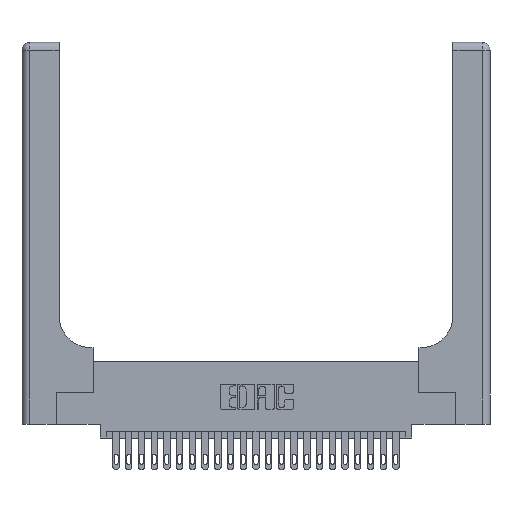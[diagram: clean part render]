
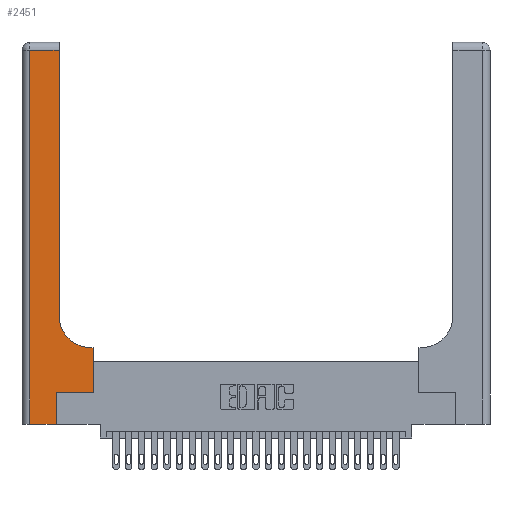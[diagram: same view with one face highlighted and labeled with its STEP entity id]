
A CAD part, top view. The second image highlights one B-rep face of the part: STEP entity #2451.
In plain terms, the highlighted planar face has unit normal (0, 0, 1).
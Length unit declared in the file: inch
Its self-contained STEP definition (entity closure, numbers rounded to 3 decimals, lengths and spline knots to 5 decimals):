
#183 = CARTESIAN_POINT ( 'NONE',  ( 0.2915, 3., 0.37 ) ) ;
#458 = VERTEX_POINT ( 'NONE', #17741 ) ;
#480 = DIRECTION ( 'NONE',  ( -1., 0., 0. ) ) ;
#827 = VERTEX_POINT ( 'NONE', #19914 ) ;
#1209 = LINE ( 'NONE', #6570, #21584 ) ;
#1299 = EDGE_CURVE ( 'NONE', #20997, #16574, #18818, .T. ) ;
#1300 = CARTESIAN_POINT ( 'NONE',  ( 0.269, 0.25, 0.37 ) ) ;
#1786 = EDGE_CURVE ( 'NONE', #13174, #24860, #15011, .T. ) ;
#1800 = ORIENTED_EDGE ( 'NONE', *, *, #9180, .T. ) ;
#2208 = CARTESIAN_POINT ( 'NONE',  ( 0.269, 0., 0.37 ) ) ;
#2451 = ADVANCED_FACE ( 'NONE', ( #9106 ), #15097, .F. ) ;
#2766 = EDGE_CURVE ( 'NONE', #15341, #827, #24637, .T. ) ;
#2952 = DIRECTION ( 'NONE',  ( 0., -1., 0. ) ) ;
#3063 = ORIENTED_EDGE ( 'NONE', *, *, #10767, .T. ) ;
#3895 = AXIS2_PLACEMENT_3D ( 'NONE', #12921, #8910, #14828 ) ;
#4445 = DIRECTION ( 'NONE',  ( 1., 0., 0. ) ) ;
#4586 = CARTESIAN_POINT ( 'NONE',  ( 0.5585, 0.25, 0.37 ) ) ;
#5791 = VERTEX_POINT ( 'NONE', #15168 ) ;
#6570 = CARTESIAN_POINT ( 'NONE',  ( 0.2915, 0.6, 0.37 ) ) ;
#6853 = EDGE_CURVE ( 'NONE', #24860, #24663, #12573, .T. ) ;
#7615 = VECTOR ( 'NONE', #8478, 39.37008 ) ;
#7775 = VECTOR ( 'NONE', #24656, 39.37008 ) ;
#8134 = LINE ( 'NONE', #23337, #17530 ) ;
#8391 = CARTESIAN_POINT ( 'NONE',  ( 0.269, 0., 0.37 ) ) ;
#8478 = DIRECTION ( 'NONE',  ( 0., 1., 0. ) ) ;
#8891 = VECTOR ( 'NONE', #2952, 39.37008 ) ;
#8910 = DIRECTION ( 'NONE',  ( 0., 0., -1. ) ) ;
#8994 = EDGE_LOOP ( 'NONE', ( #13661, #10979, #3063, #17687, #13102, #21890, #11322, #15018, #1800 ) ) ;
#9067 = LINE ( 'NONE', #15370, #24345 ) ;
#9106 = FACE_OUTER_BOUND ( 'NONE', #8994, .T. ) ;
#9180 = EDGE_CURVE ( 'NONE', #458, #15341, #24648, .T. ) ;
#9673 = DIRECTION ( 'NONE',  ( 1., 0., 0. ) ) ;
#10738 = CARTESIAN_POINT ( 'NONE',  ( 0.5585, 0.25, 0.37 ) ) ;
#10767 = EDGE_CURVE ( 'NONE', #5791, #13174, #11716, .T. ) ;
#10829 = DIRECTION ( 'NONE',  ( 0., 1., 0. ) ) ;
#10979 = ORIENTED_EDGE ( 'NONE', *, *, #14374, .T. ) ;
#11322 = ORIENTED_EDGE ( 'NONE', *, *, #1299, .T. ) ;
#11393 = DIRECTION ( 'NONE',  ( -1., 0., 0. ) ) ;
#11716 = LINE ( 'NONE', #16866, #8891 ) ;
#12047 = CARTESIAN_POINT ( 'NONE',  ( 0.06, 0., 0.37 ) ) ;
#12216 = VECTOR ( 'NONE', #10829, 39.37008 ) ;
#12573 = LINE ( 'NONE', #8391, #7615 ) ;
#12921 = CARTESIAN_POINT ( 'NONE',  ( 0., 3., 0.37 ) ) ;
#13102 = ORIENTED_EDGE ( 'NONE', *, *, #6853, .T. ) ;
#13174 = VERTEX_POINT ( 'NONE', #12047 ) ;
#13515 = AXIS2_PLACEMENT_3D ( 'NONE', #22555, #16450, #4445 ) ;
#13661 = ORIENTED_EDGE ( 'NONE', *, *, #2766, .T. ) ;
#14374 = EDGE_CURVE ( 'NONE', #827, #5791, #9067, .T. ) ;
#14589 = DIRECTION ( 'NONE',  ( 1., 0., 0. ) ) ;
#14777 = EDGE_CURVE ( 'NONE', #16574, #458, #1209, .T. ) ;
#14828 = DIRECTION ( 'NONE',  ( -1., 0., 0. ) ) ;
#15011 = LINE ( 'NONE', #15410, #24443 ) ;
#15018 = ORIENTED_EDGE ( 'NONE', *, *, #14777, .T. ) ;
#15097 = PLANE ( 'NONE',  #3895 ) ;
#15168 = CARTESIAN_POINT ( 'NONE',  ( 0.06, 2.94, 0.37 ) ) ;
#15341 = VERTEX_POINT ( 'NONE', #17788 ) ;
#15370 = CARTESIAN_POINT ( 'NONE',  ( 0., 2.94, 0.37 ) ) ;
#15410 = CARTESIAN_POINT ( 'NONE',  ( 0., 0., 0.37 ) ) ;
#16450 = DIRECTION ( 'NONE',  ( 0., 0., -1. ) ) ;
#16574 = VERTEX_POINT ( 'NONE', #19877 ) ;
#16866 = CARTESIAN_POINT ( 'NONE',  ( 0.06, 3., 0.37 ) ) ;
#17530 = VECTOR ( 'NONE', #9673, 39.37008 ) ;
#17687 = ORIENTED_EDGE ( 'NONE', *, *, #1786, .T. ) ;
#17741 = CARTESIAN_POINT ( 'NONE',  ( 0.5415, 0.6, 0.37 ) ) ;
#17788 = CARTESIAN_POINT ( 'NONE',  ( 0.2915, 0.85, 0.37 ) ) ;
#18818 = LINE ( 'NONE', #10738, #12216 ) ;
#19602 = EDGE_CURVE ( 'NONE', #24663, #20997, #8134, .T. ) ;
#19877 = CARTESIAN_POINT ( 'NONE',  ( 0.5585, 0.6, 0.37 ) ) ;
#19914 = CARTESIAN_POINT ( 'NONE',  ( 0.2915, 2.94, 0.37 ) ) ;
#20997 = VERTEX_POINT ( 'NONE', #4586 ) ;
#21584 = VECTOR ( 'NONE', #480, 39.37008 ) ;
#21890 = ORIENTED_EDGE ( 'NONE', *, *, #19602, .T. ) ;
#22555 = CARTESIAN_POINT ( 'NONE',  ( 0.5415, 0.85, 0.37 ) ) ;
#23337 = CARTESIAN_POINT ( 'NONE',  ( 0.269, 0.25, 0.37 ) ) ;
#24345 = VECTOR ( 'NONE', #11393, 39.37008 ) ;
#24443 = VECTOR ( 'NONE', #14589, 39.37008 ) ;
#24637 = LINE ( 'NONE', #183, #7775 ) ;
#24648 = CIRCLE ( 'NONE', #13515, 0.25 ) ;
#24656 = DIRECTION ( 'NONE',  ( 0., 1., 0. ) ) ;
#24663 = VERTEX_POINT ( 'NONE', #1300 ) ;
#24860 = VERTEX_POINT ( 'NONE', #2208 ) ;
